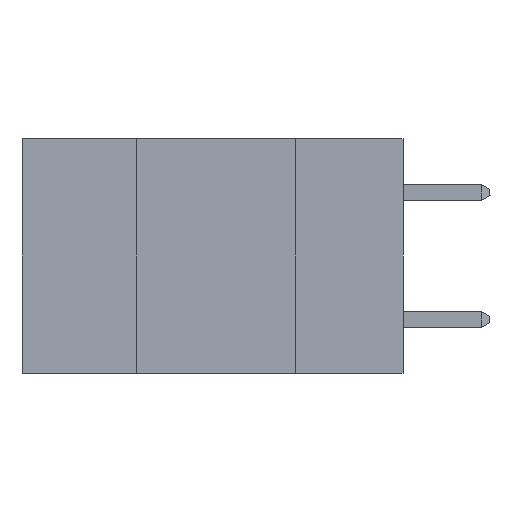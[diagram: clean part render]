
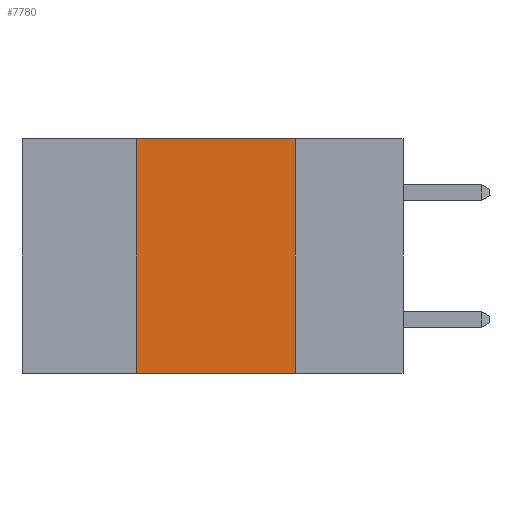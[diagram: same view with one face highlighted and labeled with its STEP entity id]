
A CAD part, left-side view. The second image highlights one B-rep face of the part: STEP entity #7780.
In plain terms, the highlighted planar face has unit normal (-1, 0, 0).
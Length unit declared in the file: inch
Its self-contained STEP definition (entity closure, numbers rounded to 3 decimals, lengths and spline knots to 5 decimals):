
#298 = ORIENTED_EDGE ( 'NONE', *, *, #3484, .F. ) ;
#1494 = EDGE_LOOP ( 'NONE', ( #298, #15239, #18798, #27578 ) ) ;
#3484 = EDGE_CURVE ( 'NONE', #16573, #7191, #29209, .T. ) ;
#4562 = CARTESIAN_POINT ( 'NONE',  ( 0., 0.6, -0.37 ) ) ;
#4684 = VERTEX_POINT ( 'NONE', #24417 ) ;
#4902 = DIRECTION ( 'NONE',  ( 0., 0., -1. ) ) ;
#4946 = VECTOR ( 'NONE', #4902, 39.37008 ) ;
#6178 = DIRECTION ( 'NONE',  ( 0., 0., 1. ) ) ;
#7191 = VERTEX_POINT ( 'NONE', #13215 ) ;
#7780 = ADVANCED_FACE ( 'NONE', ( #34500 ), #31398, .F. ) ;
#9136 = LINE ( 'NONE', #33009, #38495 ) ;
#9558 = CARTESIAN_POINT ( 'NONE',  ( 0., 0.42, 0. ) ) ;
#10807 = DIRECTION ( 'NONE',  ( 0., 0., -1. ) ) ;
#13082 = VECTOR ( 'NONE', #25518, 39.37008 ) ;
#13215 = CARTESIAN_POINT ( 'NONE',  ( 0., 0.17, -0.37 ) ) ;
#13743 = CARTESIAN_POINT ( 'NONE',  ( 0., 0.6, 0. ) ) ;
#14324 = CARTESIAN_POINT ( 'NONE',  ( 0., 0.6, 0. ) ) ;
#15239 = ORIENTED_EDGE ( 'NONE', *, *, #29200, .F. ) ;
#16573 = VERTEX_POINT ( 'NONE', #30673 ) ;
#18798 = ORIENTED_EDGE ( 'NONE', *, *, #38382, .F. ) ;
#19450 = LINE ( 'NONE', #13743, #13082 ) ;
#19641 = DIRECTION ( 'NONE',  ( 1., 0., 0. ) ) ;
#23081 = VECTOR ( 'NONE', #28478, 39.37008 ) ;
#24417 = CARTESIAN_POINT ( 'NONE',  ( 0., 0.42, -0.37 ) ) ;
#24725 = VERTEX_POINT ( 'NONE', #9558 ) ;
#25518 = DIRECTION ( 'NONE',  ( 0., -1., 0. ) ) ;
#27481 = EDGE_CURVE ( 'NONE', #4684, #7191, #34141, .T. ) ;
#27578 = ORIENTED_EDGE ( 'NONE', *, *, #27481, .T. ) ;
#28399 = AXIS2_PLACEMENT_3D ( 'NONE', #14324, #19641, #10807 ) ;
#28478 = DIRECTION ( 'NONE',  ( 0., -1., 0. ) ) ;
#29200 = EDGE_CURVE ( 'NONE', #24725, #16573, #19450, .T. ) ;
#29209 = LINE ( 'NONE', #35254, #4946 ) ;
#30673 = CARTESIAN_POINT ( 'NONE',  ( 0., 0.17, 0. ) ) ;
#31398 = PLANE ( 'NONE',  #28399 ) ;
#33009 = CARTESIAN_POINT ( 'NONE',  ( 0., 0.42, 0. ) ) ;
#34141 = LINE ( 'NONE', #4562, #23081 ) ;
#34500 = FACE_OUTER_BOUND ( 'NONE', #1494, .T. ) ;
#35254 = CARTESIAN_POINT ( 'NONE',  ( 0., 0.17, 0. ) ) ;
#38382 = EDGE_CURVE ( 'NONE', #4684, #24725, #9136, .T. ) ;
#38495 = VECTOR ( 'NONE', #6178, 39.37008 ) ;
